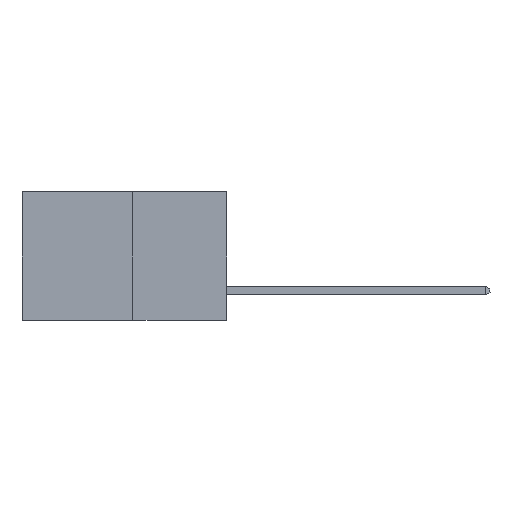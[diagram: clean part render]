
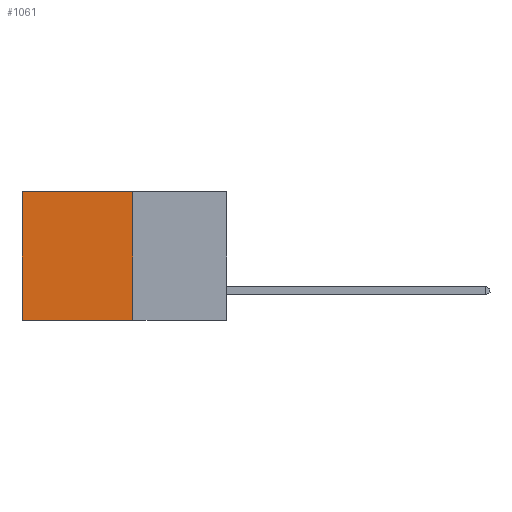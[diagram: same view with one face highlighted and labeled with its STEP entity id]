
A CAD part, left-side view. The second image highlights one B-rep face of the part: STEP entity #1061.
In plain terms, the highlighted planar face has unit normal (-1, 0, 0).
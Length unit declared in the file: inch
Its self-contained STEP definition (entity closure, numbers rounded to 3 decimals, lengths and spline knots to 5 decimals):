
#55 = EDGE_LOOP ( 'NONE', ( #9488, #6844, #8824, #7543 ) ) ;
#834 = EDGE_CURVE ( 'NONE', #2679, #7103, #9179, .T. ) ;
#1061 = ADVANCED_FACE ( 'NONE', ( #3508 ), #7431, .F. ) ;
#2132 = VECTOR ( 'NONE', #10009, 39.37008 ) ;
#2537 = CARTESIAN_POINT ( 'NONE',  ( 0.277, 0.59, -0.37 ) ) ;
#2679 = VERTEX_POINT ( 'NONE', #9128 ) ;
#3244 = VECTOR ( 'NONE', #6365, 39.37008 ) ;
#3508 = FACE_OUTER_BOUND ( 'NONE', #55, .T. ) ;
#3930 = CARTESIAN_POINT ( 'NONE',  ( 0.277, 0.27, -0.37 ) ) ;
#4022 = CARTESIAN_POINT ( 'NONE',  ( 0.277, 0.27, 0. ) ) ;
#4407 = CARTESIAN_POINT ( 'NONE',  ( 0.277, 0.27, -0.37 ) ) ;
#5067 = DIRECTION ( 'NONE',  ( 1., 0., 0. ) ) ;
#5588 = CARTESIAN_POINT ( 'NONE',  ( 0.277, 0.27, -0.37 ) ) ;
#5820 = DIRECTION ( 'NONE',  ( 0., 0., -1. ) ) ;
#5937 = CARTESIAN_POINT ( 'NONE',  ( 0.277, 0.59, -0.37 ) ) ;
#6365 = DIRECTION ( 'NONE',  ( 0., 1., 0. ) ) ;
#6453 = EDGE_CURVE ( 'NONE', #7978, #8876, #9218, .T. ) ;
#6766 = CARTESIAN_POINT ( 'NONE',  ( 0.277, 0.59, 0. ) ) ;
#6771 = EDGE_CURVE ( 'NONE', #8876, #7103, #7622, .T. ) ;
#6844 = ORIENTED_EDGE ( 'NONE', *, *, #834, .F. ) ;
#7103 = VERTEX_POINT ( 'NONE', #2537 ) ;
#7272 = VECTOR ( 'NONE', #7935, 39.37008 ) ;
#7431 = PLANE ( 'NONE',  #9223 ) ;
#7543 = ORIENTED_EDGE ( 'NONE', *, *, #6453, .T. ) ;
#7622 = LINE ( 'NONE', #5937, #9324 ) ;
#7935 = DIRECTION ( 'NONE',  ( 0., 1., 0. ) ) ;
#7978 = VERTEX_POINT ( 'NONE', #4022 ) ;
#8305 = CARTESIAN_POINT ( 'NONE',  ( 0.277, 0.27, 0. ) ) ;
#8314 = LINE ( 'NONE', #3930, #2132 ) ;
#8824 = ORIENTED_EDGE ( 'NONE', *, *, #9314, .F. ) ;
#8876 = VERTEX_POINT ( 'NONE', #6766 ) ;
#9128 = CARTESIAN_POINT ( 'NONE',  ( 0.277, 0.27, -0.37 ) ) ;
#9179 = LINE ( 'NONE', #4407, #3244 ) ;
#9218 = LINE ( 'NONE', #8305, #7272 ) ;
#9223 = AXIS2_PLACEMENT_3D ( 'NONE', #5588, #5067, #9961 ) ;
#9314 = EDGE_CURVE ( 'NONE', #7978, #2679, #8314, .T. ) ;
#9324 = VECTOR ( 'NONE', #5820, 39.37008 ) ;
#9488 = ORIENTED_EDGE ( 'NONE', *, *, #6771, .T. ) ;
#9961 = DIRECTION ( 'NONE',  ( 0., 0., -1. ) ) ;
#10009 = DIRECTION ( 'NONE',  ( 0., 0., -1. ) ) ;
